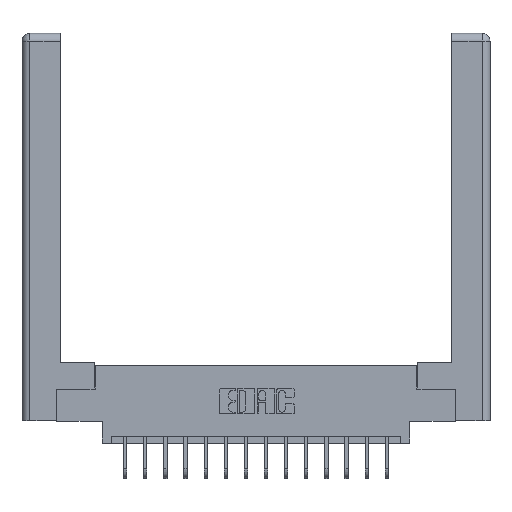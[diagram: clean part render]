
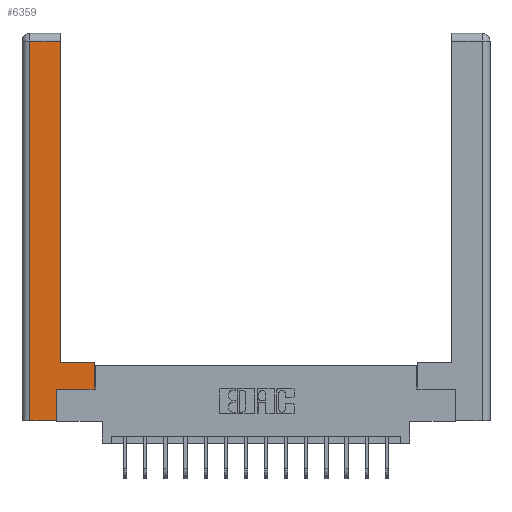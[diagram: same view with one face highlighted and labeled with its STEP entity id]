
A CAD part, top view. The second image highlights one B-rep face of the part: STEP entity #6359.
In plain terms, the highlighted planar face has unit normal (0, 0, 1).
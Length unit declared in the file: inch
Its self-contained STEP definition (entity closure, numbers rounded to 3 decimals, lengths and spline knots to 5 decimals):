
#147 = DIRECTION ( 'NONE',  ( 1., 0., 0. ) ) ;
#284 = ORIENTED_EDGE ( 'NONE', *, *, #10433, .T. ) ;
#391 = DIRECTION ( 'NONE',  ( 0., -1., 0. ) ) ;
#421 = ORIENTED_EDGE ( 'NONE', *, *, #3448, .T. ) ;
#478 = LINE ( 'NONE', #8169, #1151 ) ;
#537 = CARTESIAN_POINT ( 'NONE',  ( 0.565, 0.245, 0. ) ) ;
#591 = CARTESIAN_POINT ( 'NONE',  ( 0.295, 3., 0. ) ) ;
#1151 = VECTOR ( 'NONE', #11086, 39.37008 ) ;
#1334 = EDGE_CURVE ( 'NONE', #17834, #2105, #16554, .T. ) ;
#1989 = DIRECTION ( 'NONE',  ( -1., 0., 0. ) ) ;
#2105 = VERTEX_POINT ( 'NONE', #537 ) ;
#2433 = AXIS2_PLACEMENT_3D ( 'NONE', #14699, #7487, #16111 ) ;
#3276 = VECTOR ( 'NONE', #391, 39.37008 ) ;
#3448 = EDGE_CURVE ( 'NONE', #11119, #13753, #478, .T. ) ;
#3706 = VERTEX_POINT ( 'NONE', #12568 ) ;
#3858 = VECTOR ( 'NONE', #1989, 39.37008 ) ;
#4349 = CARTESIAN_POINT ( 'NONE',  ( 0.0615, 2.94, 0. ) ) ;
#4742 = EDGE_CURVE ( 'NONE', #13753, #7029, #15855, .T. ) ;
#5209 = VECTOR ( 'NONE', #12000, 39.37008 ) ;
#5444 = ORIENTED_EDGE ( 'NONE', *, *, #8541, .T. ) ;
#5488 = LINE ( 'NONE', #4349, #3858 ) ;
#5760 = PLANE ( 'NONE',  #2433 ) ;
#5773 = VECTOR ( 'NONE', #7049, 39.37008 ) ;
#6037 = CARTESIAN_POINT ( 'NONE',  ( 0.265, 0.245, 0. ) ) ;
#6106 = DIRECTION ( 'NONE',  ( 0., 1., 0. ) ) ;
#6248 = VECTOR ( 'NONE', #147, 39.37008 ) ;
#6359 = ADVANCED_FACE ( 'NONE', ( #7013 ), #5760, .F. ) ;
#7013 = FACE_OUTER_BOUND ( 'NONE', #12771, .T. ) ;
#7029 = VERTEX_POINT ( 'NONE', #14751 ) ;
#7049 = DIRECTION ( 'NONE',  ( 0., 1., 0. ) ) ;
#7487 = DIRECTION ( 'NONE',  ( 0., 0., -1. ) ) ;
#7562 = CARTESIAN_POINT ( 'NONE',  ( 0.265, 0., 0. ) ) ;
#8037 = VECTOR ( 'NONE', #16766, 39.37008 ) ;
#8169 = CARTESIAN_POINT ( 'NONE',  ( 0.295, 0.45, 0. ) ) ;
#8172 = CARTESIAN_POINT ( 'NONE',  ( 0.565, 0.45, 0. ) ) ;
#8352 = VERTEX_POINT ( 'NONE', #19056 ) ;
#8497 = EDGE_CURVE ( 'NONE', #17797, #17834, #9941, .T. ) ;
#8541 = EDGE_CURVE ( 'NONE', #8352, #3706, #15728, .T. ) ;
#9195 = ORIENTED_EDGE ( 'NONE', *, *, #8497, .T. ) ;
#9224 = CARTESIAN_POINT ( 'NONE',  ( 0.0615, 0., 0. ) ) ;
#9941 = LINE ( 'NONE', #6037, #17789 ) ;
#10433 = EDGE_CURVE ( 'NONE', #7029, #8352, #5488, .T. ) ;
#11086 = DIRECTION ( 'NONE',  ( -1., 0., 0. ) ) ;
#11119 = VERTEX_POINT ( 'NONE', #15869 ) ;
#12000 = DIRECTION ( 'NONE',  ( 1., 0., 0. ) ) ;
#12018 = LINE ( 'NONE', #7562, #6248 ) ;
#12568 = CARTESIAN_POINT ( 'NONE',  ( 0.0615, 0., 0. ) ) ;
#12771 = EDGE_LOOP ( 'NONE', ( #14816, #284, #5444, #13399, #9195, #16298, #13774, #421 ) ) ;
#13238 = CARTESIAN_POINT ( 'NONE',  ( 0.265, 0.245, 0. ) ) ;
#13399 = ORIENTED_EDGE ( 'NONE', *, *, #15446, .T. ) ;
#13753 = VERTEX_POINT ( 'NONE', #16937 ) ;
#13774 = ORIENTED_EDGE ( 'NONE', *, *, #18292, .T. ) ;
#14699 = CARTESIAN_POINT ( 'NONE',  ( 0., 0., 0. ) ) ;
#14751 = CARTESIAN_POINT ( 'NONE',  ( 0.295, 2.94, 0. ) ) ;
#14816 = ORIENTED_EDGE ( 'NONE', *, *, #4742, .T. ) ;
#15446 = EDGE_CURVE ( 'NONE', #3706, #17797, #12018, .T. ) ;
#15728 = LINE ( 'NONE', #9224, #3276 ) ;
#15855 = LINE ( 'NONE', #591, #8037 ) ;
#15869 = CARTESIAN_POINT ( 'NONE',  ( 0.565, 0.45, 0. ) ) ;
#16081 = CARTESIAN_POINT ( 'NONE',  ( 0.265, 0., 0. ) ) ;
#16111 = DIRECTION ( 'NONE',  ( -1., 0., 0. ) ) ;
#16298 = ORIENTED_EDGE ( 'NONE', *, *, #1334, .T. ) ;
#16554 = LINE ( 'NONE', #18802, #5209 ) ;
#16766 = DIRECTION ( 'NONE',  ( 0., 1., 0. ) ) ;
#16937 = CARTESIAN_POINT ( 'NONE',  ( 0.295, 0.45, 0. ) ) ;
#17076 = LINE ( 'NONE', #8172, #5773 ) ;
#17789 = VECTOR ( 'NONE', #6106, 39.37008 ) ;
#17797 = VERTEX_POINT ( 'NONE', #16081 ) ;
#17834 = VERTEX_POINT ( 'NONE', #13238 ) ;
#18292 = EDGE_CURVE ( 'NONE', #2105, #11119, #17076, .T. ) ;
#18802 = CARTESIAN_POINT ( 'NONE',  ( 0.565, 0.245, 0. ) ) ;
#19056 = CARTESIAN_POINT ( 'NONE',  ( 0.0615, 2.94, 0. ) ) ;
